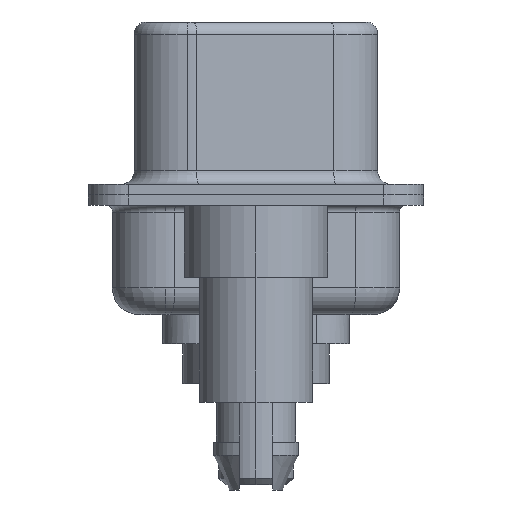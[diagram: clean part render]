
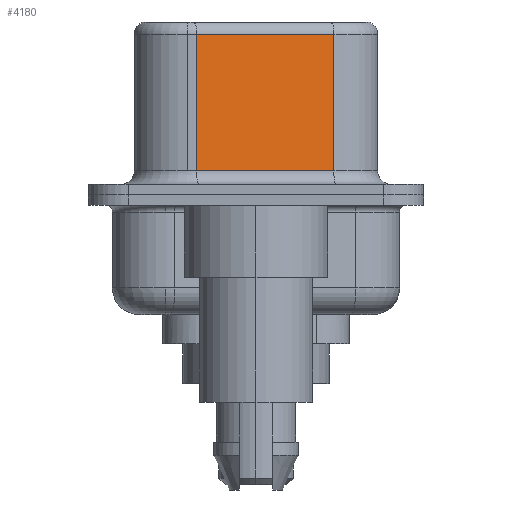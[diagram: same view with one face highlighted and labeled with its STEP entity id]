
A CAD part, left-side view. The second image highlights one B-rep face of the part: STEP entity #4180.
In plain terms, the highlighted planar face has unit normal (-0.985, -0.174, 0).
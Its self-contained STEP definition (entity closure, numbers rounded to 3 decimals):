
#352 = VECTOR ( 'NONE', #11108, 1000. ) ;
#769 = LINE ( 'NONE', #12494, #1484 ) ;
#1001 = ORIENTED_EDGE ( 'NONE', *, *, #9927, .T. ) ;
#1187 = ORIENTED_EDGE ( 'NONE', *, *, #1531, .T. ) ;
#1387 = ORIENTED_EDGE ( 'NONE', *, *, #12695, .F. ) ;
#1484 = VECTOR ( 'NONE', #5092, 1000. ) ;
#1531 = EDGE_CURVE ( 'NONE', #5282, #8164, #769, .T. ) ;
#1832 = DIRECTION ( 'NONE',  ( -0.174, 0.985, 0. ) ) ;
#1943 = DIRECTION ( 'NONE',  ( -0.174, 0.985, 0. ) ) ;
#2093 = DIRECTION ( 'NONE',  ( 0.985, 0.174, 0. ) ) ;
#2815 = VERTEX_POINT ( 'NONE', #3754 ) ;
#3238 = CARTESIAN_POINT ( 'NONE',  ( 3.675, 2.233, 6.02 ) ) ;
#3437 = VECTOR ( 'NONE', #1832, 1000. ) ;
#3754 = CARTESIAN_POINT ( 'NONE',  ( 4.585, -2.927, 6.02 ) ) ;
#3963 = CARTESIAN_POINT ( 'NONE',  ( 4.585, -2.927, 0.9 ) ) ;
#4180 = ADVANCED_FACE ( 'NONE', ( #6414 ), #6773, .F. ) ;
#4272 = VECTOR ( 'NONE', #8917, 1000. ) ;
#5092 = DIRECTION ( 'NONE',  ( 0., 0., -1. ) ) ;
#5282 = VERTEX_POINT ( 'NONE', #3238 ) ;
#6397 = CARTESIAN_POINT ( 'NONE',  ( 4.585, -2.927, 0.9 ) ) ;
#6414 = FACE_OUTER_BOUND ( 'NONE', #8355, .T. ) ;
#6773 = PLANE ( 'NONE',  #14124 ) ;
#6994 = LINE ( 'NONE', #3963, #352 ) ;
#7634 = EDGE_CURVE ( 'NONE', #8164, #12354, #6994, .T. ) ;
#8164 = VERTEX_POINT ( 'NONE', #11227 ) ;
#8186 = ORIENTED_EDGE ( 'NONE', *, *, #7634, .T. ) ;
#8355 = EDGE_LOOP ( 'NONE', ( #1387, #1001, #1187, #8186 ) ) ;
#8917 = DIRECTION ( 'NONE',  ( 0., 0., -1. ) ) ;
#9732 = LINE ( 'NONE', #10100, #3437 ) ;
#9927 = EDGE_CURVE ( 'NONE', #2815, #5282, #9732, .T. ) ;
#10100 = CARTESIAN_POINT ( 'NONE',  ( 4.585, -2.927, 6.02 ) ) ;
#11108 = DIRECTION ( 'NONE',  ( 0.174, -0.985, 0. ) ) ;
#11227 = CARTESIAN_POINT ( 'NONE',  ( 3.675, 2.233, 0.9 ) ) ;
#12354 = VERTEX_POINT ( 'NONE', #6397 ) ;
#12439 = CARTESIAN_POINT ( 'NONE',  ( 4.585, -2.927, 6.52 ) ) ;
#12494 = CARTESIAN_POINT ( 'NONE',  ( 3.675, 2.233, 6.52 ) ) ;
#12695 = EDGE_CURVE ( 'NONE', #2815, #12354, #14051, .T. ) ;
#13763 = CARTESIAN_POINT ( 'NONE',  ( 4.585, -2.927, 6.52 ) ) ;
#14051 = LINE ( 'NONE', #12439, #4272 ) ;
#14124 = AXIS2_PLACEMENT_3D ( 'NONE', #13763, #2093, #1943 ) ;
